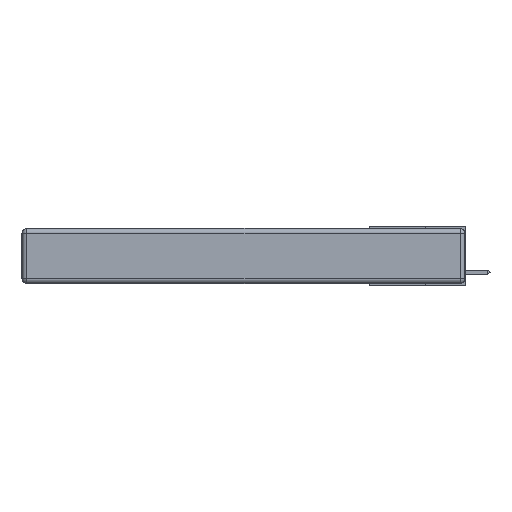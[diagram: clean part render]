
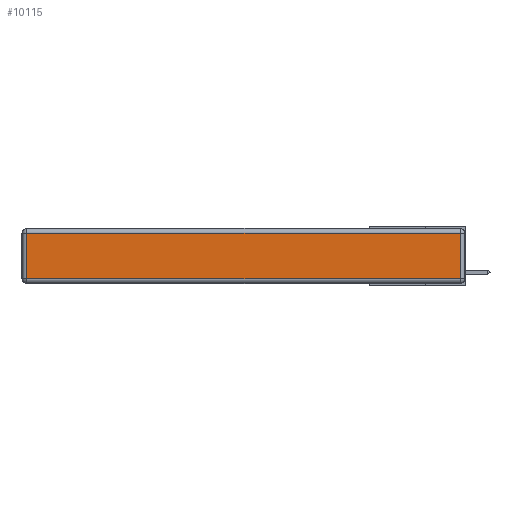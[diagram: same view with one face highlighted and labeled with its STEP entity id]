
A CAD part, left-side view. The second image highlights one B-rep face of the part: STEP entity #10115.
In plain terms, the highlighted planar face has unit normal (-1, 0, 0).
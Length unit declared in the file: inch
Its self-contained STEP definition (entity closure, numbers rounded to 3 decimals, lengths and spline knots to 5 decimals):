
#418 = EDGE_CURVE ( 'NONE', #13892, #13501, #14832, .T. ) ;
#513 = EDGE_CURVE ( 'NONE', #13501, #4122, #7685, .T. ) ;
#1301 = VERTEX_POINT ( 'NONE', #15760 ) ;
#2947 = EDGE_CURVE ( 'NONE', #4122, #1301, #9168, .T. ) ;
#3074 = EDGE_CURVE ( 'NONE', #1301, #13892, #4684, .T. ) ;
#3599 = DIRECTION ( 'NONE',  ( 0., 0., -1. ) ) ;
#3825 = DIRECTION ( 'NONE',  ( -1., 0., 0. ) ) ;
#3933 = PLANE ( 'NONE',  #8837 ) ;
#4122 = VERTEX_POINT ( 'NONE', #14751 ) ;
#4684 = LINE ( 'NONE', #5787, #11021 ) ;
#5758 = VECTOR ( 'NONE', #12537, 39.37008 ) ;
#5787 = CARTESIAN_POINT ( 'NONE',  ( 0., 2.75, -0.03 ) ) ;
#7663 = ORIENTED_EDGE ( 'NONE', *, *, #418, .T. ) ;
#7685 = LINE ( 'NONE', #13382, #8968 ) ;
#8478 = EDGE_LOOP ( 'NONE', ( #12487, #9135, #17153, #7663 ) ) ;
#8837 = AXIS2_PLACEMENT_3D ( 'NONE', #16046, #3825, #13440 ) ;
#8968 = VECTOR ( 'NONE', #10616, 39.37008 ) ;
#9071 = CARTESIAN_POINT ( 'NONE',  ( 0., 2.72, -0.03 ) ) ;
#9135 = ORIENTED_EDGE ( 'NONE', *, *, #2947, .T. ) ;
#9168 = LINE ( 'NONE', #9853, #5758 ) ;
#9853 = CARTESIAN_POINT ( 'NONE',  ( 0., 0.03, -0.343 ) ) ;
#9919 = DIRECTION ( 'NONE',  ( 0., 1., 0. ) ) ;
#10115 = ADVANCED_FACE ( 'NONE', ( #14387 ), #3933, .T. ) ;
#10616 = DIRECTION ( 'NONE',  ( 0., -1., 0. ) ) ;
#11021 = VECTOR ( 'NONE', #9919, 39.37008 ) ;
#11580 = CARTESIAN_POINT ( 'NONE',  ( 0., 2.72, -0.313 ) ) ;
#12487 = ORIENTED_EDGE ( 'NONE', *, *, #513, .T. ) ;
#12537 = DIRECTION ( 'NONE',  ( 0., 0., 1. ) ) ;
#13382 = CARTESIAN_POINT ( 'NONE',  ( 0., 0., -0.313 ) ) ;
#13440 = DIRECTION ( 'NONE',  ( 0., 0., 1. ) ) ;
#13501 = VERTEX_POINT ( 'NONE', #11580 ) ;
#13581 = VECTOR ( 'NONE', #3599, 39.37008 ) ;
#13892 = VERTEX_POINT ( 'NONE', #9071 ) ;
#14321 = CARTESIAN_POINT ( 'NONE',  ( 0., 2.72, -0.343 ) ) ;
#14387 = FACE_OUTER_BOUND ( 'NONE', #8478, .T. ) ;
#14751 = CARTESIAN_POINT ( 'NONE',  ( 0., 0.03, -0.313 ) ) ;
#14832 = LINE ( 'NONE', #14321, #13581 ) ;
#15760 = CARTESIAN_POINT ( 'NONE',  ( 0., 0.03, -0.03 ) ) ;
#16046 = CARTESIAN_POINT ( 'NONE',  ( 0., 0., -0.343 ) ) ;
#17153 = ORIENTED_EDGE ( 'NONE', *, *, #3074, .T. ) ;
